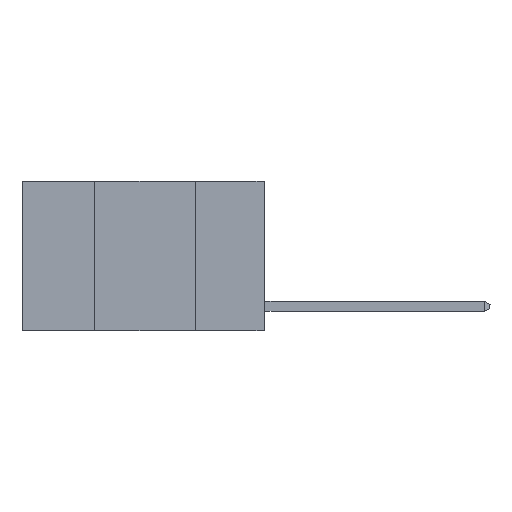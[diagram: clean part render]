
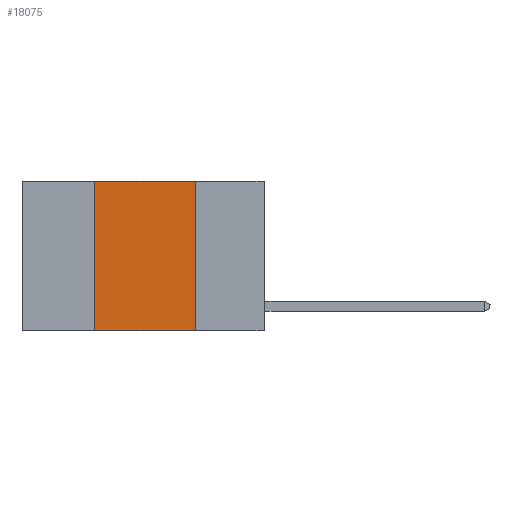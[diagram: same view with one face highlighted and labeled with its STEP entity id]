
A CAD part, left-side view. The second image highlights one B-rep face of the part: STEP entity #18075.
In plain terms, the highlighted planar face has unit normal (-1, 0, 0).
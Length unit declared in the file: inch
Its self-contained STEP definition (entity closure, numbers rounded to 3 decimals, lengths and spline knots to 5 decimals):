
#523 = EDGE_CURVE ( 'NONE', #20838, #20839, #18755, .T. ) ;
#2370 = DIRECTION ( 'NONE',  ( 0., 0., 1. ) ) ;
#3101 = VECTOR ( 'NONE', #2370, 39.37008 ) ;
#3277 = VECTOR ( 'NONE', #10855, 39.37008 ) ;
#3930 = ORIENTED_EDGE ( 'NONE', *, *, #15350, .T. ) ;
#4243 = CARTESIAN_POINT ( 'NONE',  ( 0., 0.6, 0. ) ) ;
#4246 = VERTEX_POINT ( 'NONE', #6154 ) ;
#4623 = FACE_OUTER_BOUND ( 'NONE', #8446, .T. ) ;
#4716 = CARTESIAN_POINT ( 'NONE',  ( 0., 0.17, 0. ) ) ;
#5668 = ORIENTED_EDGE ( 'NONE', *, *, #6178, .F. ) ;
#5851 = PLANE ( 'NONE',  #11971 ) ;
#6154 = CARTESIAN_POINT ( 'NONE',  ( 0., 0.42, -0.37 ) ) ;
#6178 = EDGE_CURVE ( 'NONE', #20839, #6353, #11906, .T. ) ;
#6353 = VERTEX_POINT ( 'NONE', #19482 ) ;
#6937 = DIRECTION ( 'NONE',  ( 0., -1., 0. ) ) ;
#8446 = EDGE_LOOP ( 'NONE', ( #5668, #10443, #14777, #3930 ) ) ;
#9084 = DIRECTION ( 'NONE',  ( 0., 0., -1. ) ) ;
#10443 = ORIENTED_EDGE ( 'NONE', *, *, #523, .F. ) ;
#10855 = DIRECTION ( 'NONE',  ( 0., 0., -1. ) ) ;
#11145 = CARTESIAN_POINT ( 'NONE',  ( 0., 0.42, 0. ) ) ;
#11732 = LINE ( 'NONE', #15318, #3101 ) ;
#11906 = LINE ( 'NONE', #20452, #3277 ) ;
#11971 = AXIS2_PLACEMENT_3D ( 'NONE', #17075, #18704, #9084 ) ;
#13024 = VECTOR ( 'NONE', #19424, 39.37008 ) ;
#14777 = ORIENTED_EDGE ( 'NONE', *, *, #14880, .F. ) ;
#14880 = EDGE_CURVE ( 'NONE', #4246, #20838, #11732, .T. ) ;
#15318 = CARTESIAN_POINT ( 'NONE',  ( 0., 0.42, 0. ) ) ;
#15350 = EDGE_CURVE ( 'NONE', #4246, #6353, #15697, .T. ) ;
#15697 = LINE ( 'NONE', #16571, #20443 ) ;
#16571 = CARTESIAN_POINT ( 'NONE',  ( 0., 0.6, -0.37 ) ) ;
#17075 = CARTESIAN_POINT ( 'NONE',  ( 0., 0.6, 0. ) ) ;
#18075 = ADVANCED_FACE ( 'NONE', ( #4623 ), #5851, .F. ) ;
#18704 = DIRECTION ( 'NONE',  ( 1., 0., 0. ) ) ;
#18755 = LINE ( 'NONE', #4243, #13024 ) ;
#19424 = DIRECTION ( 'NONE',  ( 0., -1., 0. ) ) ;
#19482 = CARTESIAN_POINT ( 'NONE',  ( 0., 0.17, -0.37 ) ) ;
#20443 = VECTOR ( 'NONE', #6937, 39.37008 ) ;
#20452 = CARTESIAN_POINT ( 'NONE',  ( 0., 0.17, 0. ) ) ;
#20838 = VERTEX_POINT ( 'NONE', #11145 ) ;
#20839 = VERTEX_POINT ( 'NONE', #4716 ) ;
